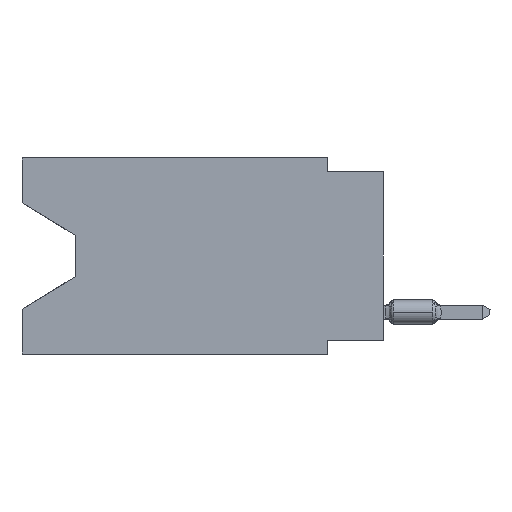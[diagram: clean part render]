
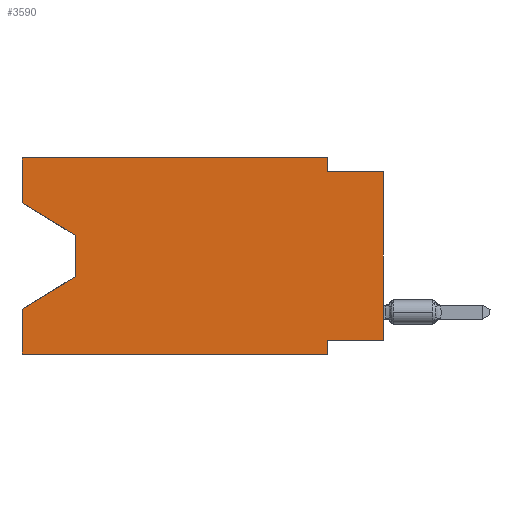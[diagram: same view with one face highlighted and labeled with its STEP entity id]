
A CAD part, left-side view. The second image highlights one B-rep face of the part: STEP entity #3590.
In plain terms, the highlighted planar face has unit normal (-1, 0, 0).
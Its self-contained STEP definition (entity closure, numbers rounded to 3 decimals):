
#139 = DIRECTION ( 'NONE',  ( 0., 0., 1. ) ) ;
#2807 = LINE ( 'NONE', #33089, #29020 ) ;
#3267 = FACE_OUTER_BOUND ( 'NONE', #20986, .T. ) ;
#3318 = DIRECTION ( 'NONE',  ( 0., -0.855, -0.519 ) ) ;
#3590 = ADVANCED_FACE ( 'NONE', ( #3267 ), #10247, .F. ) ;
#4032 = CARTESIAN_POINT ( 'NONE',  ( 0., 0., -0.635 ) ) ;
#4480 = VECTOR ( 'NONE', #21961, 1000. ) ;
#4496 = EDGE_CURVE ( 'NONE', #19972, #13969, #25269, .T. ) ;
#4778 = EDGE_CURVE ( 'NONE', #46164, #22042, #20212, .T. ) ;
#4818 = DIRECTION ( 'NONE',  ( 0., 1., 0. ) ) ;
#5059 = EDGE_CURVE ( 'NONE', #36591, #13299, #41233, .T. ) ;
#6024 = VERTEX_POINT ( 'NONE', #4032 ) ;
#8311 = CARTESIAN_POINT ( 'NONE',  ( 0., 16.383, 0. ) ) ;
#8368 = CARTESIAN_POINT ( 'NONE',  ( 0., 2.54, 0. ) ) ;
#8834 = DIRECTION ( 'NONE',  ( 0., 0., -1. ) ) ;
#9355 = LINE ( 'NONE', #34122, #39397 ) ;
#9887 = CARTESIAN_POINT ( 'NONE',  ( 0., 13.97, -3.505 ) ) ;
#10225 = DIRECTION ( 'NONE',  ( 0., -1., 0. ) ) ;
#10247 = PLANE ( 'NONE',  #24760 ) ;
#10586 = CARTESIAN_POINT ( 'NONE',  ( 0., 0., -0.635 ) ) ;
#11040 = ORIENTED_EDGE ( 'NONE', *, *, #5059, .T. ) ;
#11455 = CARTESIAN_POINT ( 'NONE',  ( 0., 0., -8.255 ) ) ;
#11977 = ORIENTED_EDGE ( 'NONE', *, *, #24269, .T. ) ;
#12575 = CARTESIAN_POINT ( 'NONE',  ( 0., 16.383, -8.89 ) ) ;
#12982 = VECTOR ( 'NONE', #3318, 1000. ) ;
#13299 = VERTEX_POINT ( 'NONE', #28852 ) ;
#13915 = DIRECTION ( 'NONE',  ( 0., 0., -1. ) ) ;
#13969 = VERTEX_POINT ( 'NONE', #47187 ) ;
#14525 = LINE ( 'NONE', #29177, #4480 ) ;
#14672 = DIRECTION ( 'NONE',  ( 0., -1., 0. ) ) ;
#14950 = CARTESIAN_POINT ( 'NONE',  ( 0., 2.54, -8.89 ) ) ;
#15080 = VECTOR ( 'NONE', #13915, 1000. ) ;
#15244 = ORIENTED_EDGE ( 'NONE', *, *, #30340, .T. ) ;
#15573 = ORIENTED_EDGE ( 'NONE', *, *, #4778, .F. ) ;
#15624 = VECTOR ( 'NONE', #4818, 1000. ) ;
#17262 = VERTEX_POINT ( 'NONE', #12575 ) ;
#17693 = EDGE_CURVE ( 'NONE', #17262, #13299, #2807, .T. ) ;
#17721 = VECTOR ( 'NONE', #14672, 1000. ) ;
#17821 = LINE ( 'NONE', #10586, #17721 ) ;
#19972 = VERTEX_POINT ( 'NONE', #8311 ) ;
#20212 = LINE ( 'NONE', #27178, #15624 ) ;
#20986 = EDGE_LOOP ( 'NONE', ( #42243, #15244, #11040, #41143, #11977, #32385, #15573, #27432, #39814, #43310, #33150, #39954 ) ) ;
#21961 = DIRECTION ( 'NONE',  ( 0., 0., 1. ) ) ;
#22042 = VERTEX_POINT ( 'NONE', #44233 ) ;
#22853 = EDGE_CURVE ( 'NONE', #46164, #6024, #14525, .T. ) ;
#24118 = VECTOR ( 'NONE', #45075, 1000. ) ;
#24269 = EDGE_CURVE ( 'NONE', #17262, #46003, #40239, .T. ) ;
#24760 = AXIS2_PLACEMENT_3D ( 'NONE', #36207, #32606, #43640 ) ;
#25269 = LINE ( 'NONE', #46665, #43229 ) ;
#26239 = DIRECTION ( 'NONE',  ( 0., 0., -1. ) ) ;
#26632 = LINE ( 'NONE', #8368, #31471 ) ;
#27149 = CARTESIAN_POINT ( 'NONE',  ( 0., 2.54, -8.89 ) ) ;
#27178 = CARTESIAN_POINT ( 'NONE',  ( 0., 0., -8.255 ) ) ;
#27432 = ORIENTED_EDGE ( 'NONE', *, *, #22853, .T. ) ;
#27557 = VECTOR ( 'NONE', #10225, 1000. ) ;
#27624 = DIRECTION ( 'NONE',  ( 0., 0., 1. ) ) ;
#28483 = VERTEX_POINT ( 'NONE', #43567 ) ;
#28852 = CARTESIAN_POINT ( 'NONE',  ( 0., 16.383, -6.852 ) ) ;
#29020 = VECTOR ( 'NONE', #139, 1000. ) ;
#29177 = CARTESIAN_POINT ( 'NONE',  ( 0., 0., 0. ) ) ;
#30340 = EDGE_CURVE ( 'NONE', #40783, #36591, #42988, .T. ) ;
#31172 = VECTOR ( 'NONE', #26239, 1000. ) ;
#31471 = VECTOR ( 'NONE', #8834, 1000. ) ;
#31761 = EDGE_CURVE ( 'NONE', #31899, #19972, #9355, .T. ) ;
#31899 = VERTEX_POINT ( 'NONE', #31948 ) ;
#31948 = CARTESIAN_POINT ( 'NONE',  ( 0., 16.383, -2.038 ) ) ;
#32385 = ORIENTED_EDGE ( 'NONE', *, *, #42954, .F. ) ;
#32606 = DIRECTION ( 'NONE',  ( 1., 0., 0. ) ) ;
#33089 = CARTESIAN_POINT ( 'NONE',  ( 0., 16.383, 0. ) ) ;
#33150 = ORIENTED_EDGE ( 'NONE', *, *, #4496, .F. ) ;
#33828 = EDGE_CURVE ( 'NONE', #28483, #6024, #17821, .T. ) ;
#34051 = CARTESIAN_POINT ( 'NONE',  ( 0., 13.97, -5.385 ) ) ;
#34122 = CARTESIAN_POINT ( 'NONE',  ( 0., 16.383, 0. ) ) ;
#36207 = CARTESIAN_POINT ( 'NONE',  ( 0., 16.383, 0. ) ) ;
#36258 = LINE ( 'NONE', #44161, #12982 ) ;
#36591 = VERTEX_POINT ( 'NONE', #45902 ) ;
#39152 = CARTESIAN_POINT ( 'NONE',  ( 0., 13.97, -3.505 ) ) ;
#39397 = VECTOR ( 'NONE', #27624, 1000. ) ;
#39814 = ORIENTED_EDGE ( 'NONE', *, *, #33828, .F. ) ;
#39954 = ORIENTED_EDGE ( 'NONE', *, *, #31761, .F. ) ;
#40239 = LINE ( 'NONE', #43611, #27557 ) ;
#40413 = LINE ( 'NONE', #14950, #31172 ) ;
#40783 = VERTEX_POINT ( 'NONE', #9887 ) ;
#41143 = ORIENTED_EDGE ( 'NONE', *, *, #17693, .F. ) ;
#41233 = LINE ( 'NONE', #34051, #24118 ) ;
#42243 = ORIENTED_EDGE ( 'NONE', *, *, #46834, .T. ) ;
#42954 = EDGE_CURVE ( 'NONE', #22042, #46003, #40413, .T. ) ;
#42988 = LINE ( 'NONE', #39152, #15080 ) ;
#43062 = DIRECTION ( 'NONE',  ( 0., -1., 0. ) ) ;
#43229 = VECTOR ( 'NONE', #43062, 1000. ) ;
#43310 = ORIENTED_EDGE ( 'NONE', *, *, #46985, .F. ) ;
#43567 = CARTESIAN_POINT ( 'NONE',  ( 0., 2.54, -0.635 ) ) ;
#43611 = CARTESIAN_POINT ( 'NONE',  ( 0., 16.383, -8.89 ) ) ;
#43640 = DIRECTION ( 'NONE',  ( 0., 0., -1. ) ) ;
#44161 = CARTESIAN_POINT ( 'NONE',  ( 0., 16.383, -2.038 ) ) ;
#44233 = CARTESIAN_POINT ( 'NONE',  ( 0., 2.54, -8.255 ) ) ;
#45075 = DIRECTION ( 'NONE',  ( 0., 0.855, -0.519 ) ) ;
#45902 = CARTESIAN_POINT ( 'NONE',  ( 0., 13.97, -5.385 ) ) ;
#46003 = VERTEX_POINT ( 'NONE', #27149 ) ;
#46164 = VERTEX_POINT ( 'NONE', #11455 ) ;
#46665 = CARTESIAN_POINT ( 'NONE',  ( 0., 16.383, 0. ) ) ;
#46834 = EDGE_CURVE ( 'NONE', #31899, #40783, #36258, .T. ) ;
#46985 = EDGE_CURVE ( 'NONE', #13969, #28483, #26632, .T. ) ;
#47187 = CARTESIAN_POINT ( 'NONE',  ( 0., 2.54, 0. ) ) ;
